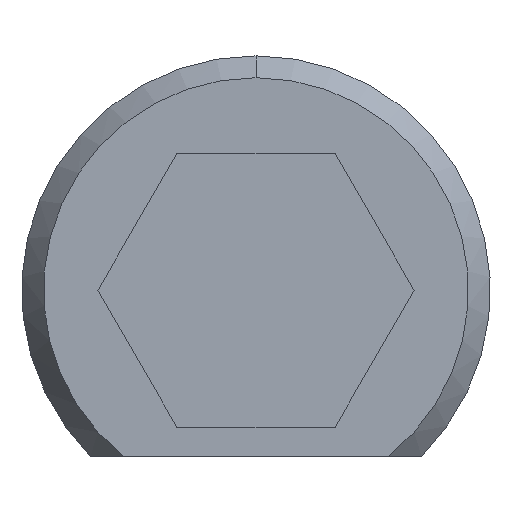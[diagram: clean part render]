
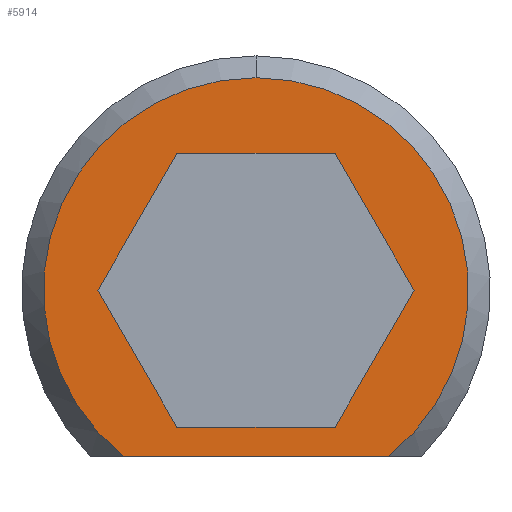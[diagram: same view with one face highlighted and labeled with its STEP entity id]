
A CAD part, front view. The second image highlights one B-rep face of the part: STEP entity #5914.
In plain terms, the highlighted planar face has unit normal (0, -1, 0).
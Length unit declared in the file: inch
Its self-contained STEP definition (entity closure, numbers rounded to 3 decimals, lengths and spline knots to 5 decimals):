
#27 = VECTOR ( 'NONE', #2917, 39.37008 ) ;
#115 = CARTESIAN_POINT ( 'NONE',  ( 0., -0.1, 0. ) ) ;
#288 = CARTESIAN_POINT ( 'NONE',  ( 0.08223, -0.1, 0.14242 ) ) ;
#295 = DIRECTION ( 'NONE',  ( 0., 0., -1. ) ) ;
#423 = DIRECTION ( 'NONE',  ( 0., 0., -1. ) ) ;
#431 = CIRCLE ( 'NONE', #1523, 0.22099 ) ;
#470 = EDGE_CURVE ( 'NONE', #5319, #7401, #6436, .T. ) ;
#521 = LINE ( 'NONE', #3699, #924 ) ;
#528 = DIRECTION ( 'NONE',  ( -0.5, 0., -0.866 ) ) ;
#647 = VECTOR ( 'NONE', #528, 39.37008 ) ;
#687 = CARTESIAN_POINT ( 'NONE',  ( 0.08223, -0.1, -0.14242 ) ) ;
#715 = EDGE_CURVE ( 'NONE', #7401, #3461, #1762, .T. ) ;
#769 = ORIENTED_EDGE ( 'NONE', *, *, #8521, .F. ) ;
#850 = CARTESIAN_POINT ( 'NONE',  ( -0.08223, -0.1, -0.14242 ) ) ;
#924 = VECTOR ( 'NONE', #3040, 39.37008 ) ;
#1039 = LINE ( 'NONE', #687, #8610 ) ;
#1153 = ORIENTED_EDGE ( 'NONE', *, *, #7279, .F. ) ;
#1238 = VERTEX_POINT ( 'NONE', #2265 ) ;
#1399 = CARTESIAN_POINT ( 'NONE',  ( 0.08223, -0.1, -0.14242 ) ) ;
#1416 = DIRECTION ( 'NONE',  ( 1., 0., 0. ) ) ;
#1523 = AXIS2_PLACEMENT_3D ( 'NONE', #6633, #7911, #423 ) ;
#1547 = DIRECTION ( 'NONE',  ( 0., -1., 0. ) ) ;
#1762 = CIRCLE ( 'NONE', #8055, 0.22099 ) ;
#1780 = EDGE_CURVE ( 'NONE', #5859, #4993, #1039, .T. ) ;
#1856 = DIRECTION ( 'NONE',  ( -0.5, 0., 0.866 ) ) ;
#1914 = ORIENTED_EDGE ( 'NONE', *, *, #715, .T. ) ;
#2172 = CARTESIAN_POINT ( 'NONE',  ( 0., -0.1, 0. ) ) ;
#2221 = FACE_OUTER_BOUND ( 'NONE', #6162, .T. ) ;
#2265 = CARTESIAN_POINT ( 'NONE',  ( 0.08223, -0.1, 0.14242 ) ) ;
#2293 = EDGE_CURVE ( 'NONE', #2341, #3797, #521, .T. ) ;
#2341 = VERTEX_POINT ( 'NONE', #4917 ) ;
#2503 = CARTESIAN_POINT ( 'NONE',  ( 0.13806, -0.1, -0.17256 ) ) ;
#2507 = VECTOR ( 'NONE', #7478, 39.37008 ) ;
#2587 = LINE ( 'NONE', #4496, #3022 ) ;
#2917 = DIRECTION ( 'NONE',  ( -1., 0., 0. ) ) ;
#3022 = VECTOR ( 'NONE', #1856, 39.37008 ) ;
#3039 = VECTOR ( 'NONE', #1416, 39.37008 ) ;
#3040 = DIRECTION ( 'NONE',  ( 0.5, 0., -0.866 ) ) ;
#3365 = ORIENTED_EDGE ( 'NONE', *, *, #1780, .F. ) ;
#3461 = VERTEX_POINT ( 'NONE', #7341 ) ;
#3684 = EDGE_CURVE ( 'NONE', #4993, #1238, #2587, .T. ) ;
#3699 = CARTESIAN_POINT ( 'NONE',  ( -0.16445, -0.1, 0. ) ) ;
#3715 = ORIENTED_EDGE ( 'NONE', *, *, #3684, .F. ) ;
#3797 = VERTEX_POINT ( 'NONE', #6683 ) ;
#3834 = ORIENTED_EDGE ( 'NONE', *, *, #470, .T. ) ;
#3915 = ORIENTED_EDGE ( 'NONE', *, *, #5017, .T. ) ;
#4203 = DIRECTION ( 'NONE',  ( 0., -1., 0. ) ) ;
#4269 = CARTESIAN_POINT ( 'NONE',  ( -0.17216, -0.1, -0.17256 ) ) ;
#4298 = PLANE ( 'NONE',  #7604 ) ;
#4441 = CARTESIAN_POINT ( 'NONE',  ( -0.08223, -0.1, 0.14242 ) ) ;
#4453 = ORIENTED_EDGE ( 'NONE', *, *, #2293, .F. ) ;
#4496 = CARTESIAN_POINT ( 'NONE',  ( 0.16445, -0.1, 0. ) ) ;
#4634 = DIRECTION ( 'NONE',  ( 0.5, 0., 0.866 ) ) ;
#4917 = CARTESIAN_POINT ( 'NONE',  ( -0.16445, -0.1, 0. ) ) ;
#4993 = VERTEX_POINT ( 'NONE', #6437 ) ;
#5017 = EDGE_CURVE ( 'NONE', #3461, #5319, #431, .T. ) ;
#5319 = VERTEX_POINT ( 'NONE', #7204 ) ;
#5541 = ORIENTED_EDGE ( 'NONE', *, *, #7940, .F. ) ;
#5829 = LINE ( 'NONE', #850, #3039 ) ;
#5859 = VERTEX_POINT ( 'NONE', #1399 ) ;
#5914 = ADVANCED_FACE ( 'NONE', ( #2221, #7505 ), #4298, .T. ) ;
#6162 = EDGE_LOOP ( 'NONE', ( #3834, #1914, #3915 ) ) ;
#6313 = EDGE_LOOP ( 'NONE', ( #1153, #5541, #3715, #3365, #769, #4453 ) ) ;
#6436 = LINE ( 'NONE', #4269, #2507 ) ;
#6437 = CARTESIAN_POINT ( 'NONE',  ( 0.16445, -0.1, 0. ) ) ;
#6633 = CARTESIAN_POINT ( 'NONE',  ( 0., -0.1, 0. ) ) ;
#6683 = CARTESIAN_POINT ( 'NONE',  ( -0.08223, -0.1, -0.14242 ) ) ;
#7074 = LINE ( 'NONE', #288, #27 ) ;
#7091 = CARTESIAN_POINT ( 'NONE',  ( -0.08223, -0.1, 0.14242 ) ) ;
#7204 = CARTESIAN_POINT ( 'NONE',  ( -0.13806, -0.1, -0.17256 ) ) ;
#7279 = EDGE_CURVE ( 'NONE', #8030, #2341, #8222, .T. ) ;
#7341 = CARTESIAN_POINT ( 'NONE',  ( 0., -0.1, 0.22099 ) ) ;
#7401 = VERTEX_POINT ( 'NONE', #2503 ) ;
#7478 = DIRECTION ( 'NONE',  ( 1., 0., 0. ) ) ;
#7505 = FACE_BOUND ( 'NONE', #6313, .T. ) ;
#7533 = DIRECTION ( 'NONE',  ( 0., 0., -1. ) ) ;
#7604 = AXIS2_PLACEMENT_3D ( 'NONE', #115, #1547, #7533 ) ;
#7911 = DIRECTION ( 'NONE',  ( 0., -1., 0. ) ) ;
#7940 = EDGE_CURVE ( 'NONE', #1238, #8030, #7074, .T. ) ;
#8030 = VERTEX_POINT ( 'NONE', #4441 ) ;
#8055 = AXIS2_PLACEMENT_3D ( 'NONE', #2172, #4203, #295 ) ;
#8222 = LINE ( 'NONE', #7091, #647 ) ;
#8521 = EDGE_CURVE ( 'NONE', #3797, #5859, #5829, .T. ) ;
#8610 = VECTOR ( 'NONE', #4634, 39.37008 ) ;
